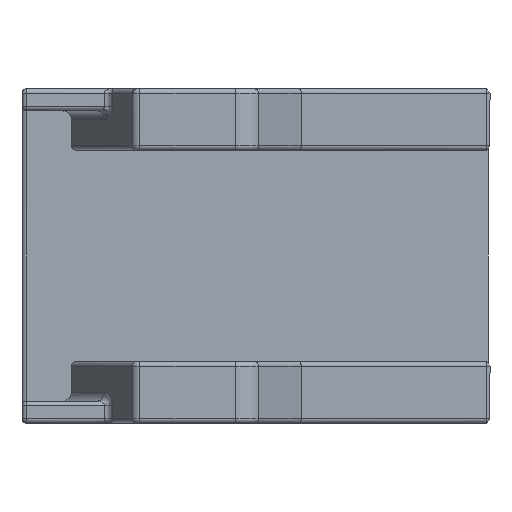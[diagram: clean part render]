
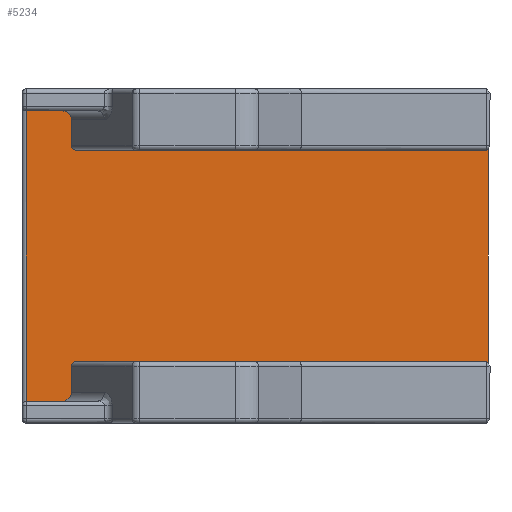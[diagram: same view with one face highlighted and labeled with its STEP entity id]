
A CAD part, left-side view. The second image highlights one B-rep face of the part: STEP entity #5234.
In plain terms, the highlighted planar face has unit normal (-1, 0, 0).
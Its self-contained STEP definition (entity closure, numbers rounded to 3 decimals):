
#726 = EDGE_CURVE ( 'NONE', #9985, #2005, #15936, .T. ) ;
#1038 = CARTESIAN_POINT ( 'NONE',  ( -82.4, -13.429, 17.5 ) ) ;
#1157 = LINE ( 'NONE', #22124, #13643 ) ;
#1219 = EDGE_CURVE ( 'NONE', #14890, #3986, #21050, .T. ) ;
#1513 = CARTESIAN_POINT ( 'NONE',  ( -82.4, -13.907, -11.5 ) ) ;
#1657 = EDGE_CURVE ( 'NONE', #3986, #16582, #3256, .T. ) ;
#1705 = CARTESIAN_POINT ( 'NONE',  ( -82.4, -13.429, -15.5 ) ) ;
#1725 = DIRECTION ( 'NONE',  ( 0., 0., -1. ) ) ;
#1759 = CARTESIAN_POINT ( 'NONE',  ( -82.4, -13.981, 13.223 ) ) ;
#1843 = CARTESIAN_POINT ( 'NONE',  ( -82.4, -61.271, 1. ) ) ;
#1848 = CARTESIAN_POINT ( 'NONE',  ( -82.4, -8.79, 1. ) ) ;
#2005 = VERTEX_POINT ( 'NONE', #19959 ) ;
#2050 = CARTESIAN_POINT ( 'NONE',  ( -82.4, -61.271, -11.4 ) ) ;
#2085 = EDGE_CURVE ( 'NONE', #19211, #19601, #5928, .T. ) ;
#2124 = LINE ( 'NONE', #9717, #24396 ) ;
#2456 = B_SPLINE_CURVE_WITH_KNOTS ( 'NONE', 3,
 ( #20971, #13055, #1759, #20611, #3974, #3623 ),
 .UNSPECIFIED., .F., .F.,
 ( 4, 2, 4 ),
 ( 0., 0., 0.001 ),
 .UNSPECIFIED. ) ;
#2497 = CARTESIAN_POINT ( 'NONE',  ( -82.4, -35.03, 17.5 ) ) ;
#2570 = CARTESIAN_POINT ( 'NONE',  ( -82.4, -61.271, 13.4 ) ) ;
#2574 = DIRECTION ( 'NONE',  ( 0., 0., 1. ) ) ;
#3256 =( BOUNDED_CURVE ( )  B_SPLINE_CURVE ( 3, ( #4893, #6760, #1038, #12588 ),
 .UNSPECIFIED., .F., .F. ) 
 B_SPLINE_CURVE_WITH_KNOTS ( ( 4, 4 ),
 ( 0., 1.571 ),
 .UNSPECIFIED. ) 
 CURVE ( )  GEOMETRIC_REPRESENTATION_ITEM ( )  RATIONAL_B_SPLINE_CURVE ( ( 1., 0.805, 0.805, 1. ) ) 
 REPRESENTATION_ITEM ( '' )  );
#3575 = CARTESIAN_POINT ( 'NONE',  ( -82.4, -12.753, -15.5 ) ) ;
#3623 = CARTESIAN_POINT ( 'NONE',  ( -82.4, -14.485, 13. ) ) ;
#3763 = VECTOR ( 'NONE', #2574, 1000. ) ;
#3878 = DIRECTION ( 'NONE',  ( 0., -1., 0. ) ) ;
#3974 = CARTESIAN_POINT ( 'NONE',  ( -82.4, -14.342, 13. ) ) ;
#3986 = VERTEX_POINT ( 'NONE', #11225 ) ;
#4193 = EDGE_CURVE ( 'NONE', #18242, #13598, #11696, .T. ) ;
#4486 = CARTESIAN_POINT ( 'NONE',  ( -82.4, -61.271, -11.4 ) ) ;
#4730 = ORIENTED_EDGE ( 'NONE', *, *, #24346, .T. ) ;
#4865 = CARTESIAN_POINT ( 'NONE',  ( -82.4, -14.413, -11. ) ) ;
#4893 = CARTESIAN_POINT ( 'NONE',  ( -82.4, -13.907, 16.5 ) ) ;
#4998 = CARTESIAN_POINT ( 'NONE',  ( -82.4, -14.344, -11.011 ) ) ;
#5045 = ORIENTED_EDGE ( 'NONE', *, *, #10420, .T. ) ;
#5196 = VERTEX_POINT ( 'NONE', #13809 ) ;
#5204 = DIRECTION ( 'NONE',  ( 0., 0., -1. ) ) ;
#5234 = ADVANCED_FACE ( 'NONE', ( #10836 ), #12434, .T. ) ;
#5490 = EDGE_CURVE ( 'NONE', #14890, #5196, #2456, .T. ) ;
#5928 = LINE ( 'NONE', #1848, #10957 ) ;
#6121 = DIRECTION ( 'NONE',  ( 0., 0.708, -0.706 ) ) ;
#6760 = CARTESIAN_POINT ( 'NONE',  ( -82.4, -13.907, 17.086 ) ) ;
#6969 = VERTEX_POINT ( 'NONE', #12746 ) ;
#6979 = CARTESIAN_POINT ( 'NONE',  ( -82.4, -14.485, -11. ) ) ;
#6993 = CARTESIAN_POINT ( 'NONE',  ( -82.4, -35.03, -11. ) ) ;
#7345 = CARTESIAN_POINT ( 'NONE',  ( -82.4, -13.907, -11.5 ) ) ;
#7756 = LINE ( 'NONE', #11953, #12028 ) ;
#7773 = DIRECTION ( 'NONE',  ( 0., 0.708, 0.706 ) ) ;
#7830 = VECTOR ( 'NONE', #23430, 1000. ) ;
#7844 = VERTEX_POINT ( 'NONE', #18092 ) ;
#8426 = LINE ( 'NONE', #1843, #9458 ) ;
#8741 = DIRECTION ( 'NONE',  ( 0., 0., 1. ) ) ;
#8966 = DIRECTION ( 'NONE',  ( -1., 0., 0. ) ) ;
#9227 = EDGE_CURVE ( 'NONE', #6969, #5196, #22511, .T. ) ;
#9271 = CARTESIAN_POINT ( 'NONE',  ( -82.4, -13.907, -15.086 ) ) ;
#9273 = ORIENTED_EDGE ( 'NONE', *, *, #5490, .F. ) ;
#9318 = AXIS2_PLACEMENT_3D ( 'NONE', #16547, #8966, #10720 ) ;
#9348 = LINE ( 'NONE', #6993, #13252 ) ;
#9458 = VECTOR ( 'NONE', #5204, 1000. ) ;
#9717 = CARTESIAN_POINT ( 'NONE',  ( -82.4, -35.03, -15.5 ) ) ;
#9985 = VERTEX_POINT ( 'NONE', #12483 ) ;
#10118 = LINE ( 'NONE', #2050, #18559 ) ;
#10172 = ORIENTED_EDGE ( 'NONE', *, *, #21109, .F. ) ;
#10228 = CARTESIAN_POINT ( 'NONE',  ( -82.4, -12.753, 17.5 ) ) ;
#10289 = ORIENTED_EDGE ( 'NONE', *, *, #13044, .F. ) ;
#10420 = EDGE_CURVE ( 'NONE', #19601, #9985, #2124, .T. ) ;
#10462 = CARTESIAN_POINT ( 'NONE',  ( -82.4, -8.79, -15.5 ) ) ;
#10720 = DIRECTION ( 'NONE',  ( 0., 0., 1. ) ) ;
#10836 = FACE_OUTER_BOUND ( 'NONE', #17031, .T. ) ;
#10917 = ORIENTED_EDGE ( 'NONE', *, *, #2085, .T. ) ;
#10957 = VECTOR ( 'NONE', #1725, 1000. ) ;
#11225 = CARTESIAN_POINT ( 'NONE',  ( -82.4, -13.907, 16.5 ) ) ;
#11696 = B_SPLINE_CURVE_WITH_KNOTS ( 'NONE', 3,
 ( #6979, #4865, #4998, #12560, #24078, #14668, #12310, #1513 ),
 .UNSPECIFIED., .F., .F.,
 ( 4, 2, 2, 4 ),
 ( 0., 0., 0., 0.001 ),
 .UNSPECIFIED. ) ;
#11920 = ORIENTED_EDGE ( 'NONE', *, *, #726, .T. ) ;
#11953 = CARTESIAN_POINT ( 'NONE',  ( -82.4, -61.271, 13.4 ) ) ;
#12028 = VECTOR ( 'NONE', #6121, 1000. ) ;
#12310 = CARTESIAN_POINT ( 'NONE',  ( -82.4, -13.907, -11.357 ) ) ;
#12434 = PLANE ( 'NONE',  #9318 ) ;
#12483 = CARTESIAN_POINT ( 'NONE',  ( -82.4, -12.753, -15.5 ) ) ;
#12560 = CARTESIAN_POINT ( 'NONE',  ( -82.4, -14.21, -11.056 ) ) ;
#12588 = CARTESIAN_POINT ( 'NONE',  ( -82.4, -12.753, 17.5 ) ) ;
#12746 = CARTESIAN_POINT ( 'NONE',  ( -82.4, -60.869, 13. ) ) ;
#13044 = EDGE_CURVE ( 'NONE', #24512, #7844, #10118, .T. ) ;
#13055 = CARTESIAN_POINT ( 'NONE',  ( -82.4, -13.907, 13.357 ) ) ;
#13252 = VECTOR ( 'NONE', #18401, 1000. ) ;
#13274 = CARTESIAN_POINT ( 'NONE',  ( -82.4, -8.79, 17.5 ) ) ;
#13598 = VERTEX_POINT ( 'NONE', #7345 ) ;
#13643 = VECTOR ( 'NONE', #8741, 1000. ) ;
#13809 = CARTESIAN_POINT ( 'NONE',  ( -82.4, -14.485, 13. ) ) ;
#13847 = ORIENTED_EDGE ( 'NONE', *, *, #16774, .T. ) ;
#14436 = ORIENTED_EDGE ( 'NONE', *, *, #9227, .T. ) ;
#14668 = CARTESIAN_POINT ( 'NONE',  ( -82.4, -13.982, -11.222 ) ) ;
#14713 = DIRECTION ( 'NONE',  ( 0., 1., 0. ) ) ;
#14890 = VERTEX_POINT ( 'NONE', #19334 ) ;
#15536 = ORIENTED_EDGE ( 'NONE', *, *, #4193, .F. ) ;
#15936 =( BOUNDED_CURVE ( )  B_SPLINE_CURVE ( 3, ( #3575, #1705, #9271, #24385 ),
 .UNSPECIFIED., .F., .T. ) 
 B_SPLINE_CURVE_WITH_KNOTS ( ( 4, 4 ),
 ( 1.571, 3.142 ),
 .UNSPECIFIED. ) 
 CURVE ( )  GEOMETRIC_REPRESENTATION_ITEM ( )  RATIONAL_B_SPLINE_CURVE ( ( 1., 0.805, 0.805, 1. ) ) 
 REPRESENTATION_ITEM ( '' )  );
#16442 = EDGE_CURVE ( 'NONE', #21294, #6969, #7756, .T. ) ;
#16547 = CARTESIAN_POINT ( 'NONE',  ( -82.4, -61.281, -15.51 ) ) ;
#16582 = VERTEX_POINT ( 'NONE', #10228 ) ;
#16708 = CARTESIAN_POINT ( 'NONE',  ( -82.4, -35.03, 13. ) ) ;
#16774 = EDGE_CURVE ( 'NONE', #18242, #7844, #9348, .T. ) ;
#16937 = ORIENTED_EDGE ( 'NONE', *, *, #1219, .T. ) ;
#17031 = EDGE_LOOP ( 'NONE', ( #13847, #10289, #10172, #18919, #14436, #9273, #16937, #23289, #23901, #10917, #5045, #11920, #4730, #15536 ) ) ;
#18092 = CARTESIAN_POINT ( 'NONE',  ( -82.4, -60.869, -11. ) ) ;
#18242 = VERTEX_POINT ( 'NONE', #21941 ) ;
#18401 = DIRECTION ( 'NONE',  ( 0., -1., 0. ) ) ;
#18559 = VECTOR ( 'NONE', #7773, 1000. ) ;
#18919 = ORIENTED_EDGE ( 'NONE', *, *, #16442, .T. ) ;
#19211 = VERTEX_POINT ( 'NONE', #13274 ) ;
#19334 = CARTESIAN_POINT ( 'NONE',  ( -82.4, -13.907, 13.5 ) ) ;
#19557 = CARTESIAN_POINT ( 'NONE',  ( -82.4, -13.907, 1. ) ) ;
#19601 = VERTEX_POINT ( 'NONE', #10462 ) ;
#19871 = EDGE_CURVE ( 'NONE', #16582, #19211, #21093, .T. ) ;
#19959 = CARTESIAN_POINT ( 'NONE',  ( -82.4, -13.907, -14.5 ) ) ;
#20611 = CARTESIAN_POINT ( 'NONE',  ( -82.4, -14.201, 13.045 ) ) ;
#20813 = VECTOR ( 'NONE', #14713, 1000. ) ;
#20971 = CARTESIAN_POINT ( 'NONE',  ( -82.4, -13.907, 13.5 ) ) ;
#21050 = LINE ( 'NONE', #19557, #3763 ) ;
#21093 = LINE ( 'NONE', #2497, #7830 ) ;
#21109 = EDGE_CURVE ( 'NONE', #21294, #24512, #8426, .T. ) ;
#21294 = VERTEX_POINT ( 'NONE', #2570 ) ;
#21941 = CARTESIAN_POINT ( 'NONE',  ( -82.4, -14.485, -11. ) ) ;
#22124 = CARTESIAN_POINT ( 'NONE',  ( -82.4, -13.907, 1. ) ) ;
#22511 = LINE ( 'NONE', #16708, #20813 ) ;
#23289 = ORIENTED_EDGE ( 'NONE', *, *, #1657, .T. ) ;
#23430 = DIRECTION ( 'NONE',  ( 0., 1., 0. ) ) ;
#23901 = ORIENTED_EDGE ( 'NONE', *, *, #19871, .T. ) ;
#24078 = CARTESIAN_POINT ( 'NONE',  ( -82.4, -14.147, -11.089 ) ) ;
#24346 = EDGE_CURVE ( 'NONE', #2005, #13598, #1157, .T. ) ;
#24385 = CARTESIAN_POINT ( 'NONE',  ( -82.4, -13.907, -14.5 ) ) ;
#24396 = VECTOR ( 'NONE', #3878, 1000. ) ;
#24512 = VERTEX_POINT ( 'NONE', #4486 ) ;
